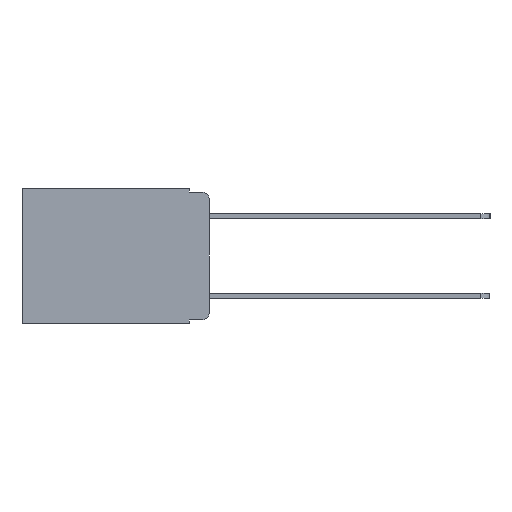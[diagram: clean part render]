
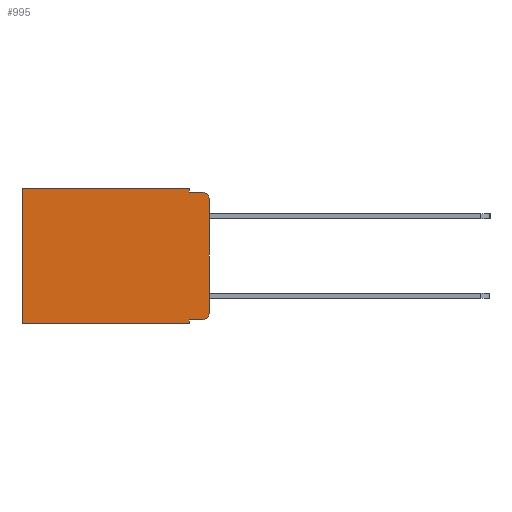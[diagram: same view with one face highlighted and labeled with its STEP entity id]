
A CAD part, left-side view. The second image highlights one B-rep face of the part: STEP entity #995.
In plain terms, the highlighted planar face has unit normal (-1, 0, 0).
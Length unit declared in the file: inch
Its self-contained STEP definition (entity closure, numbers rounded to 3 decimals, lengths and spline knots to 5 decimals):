
#72 = LINE ( 'NONE', #1308, #7037 ) ;
#288 = DIRECTION ( 'NONE',  ( 0., 0., -1. ) ) ;
#487 = CARTESIAN_POINT ( 'NONE',  ( 0.298, 0.051, 0. ) ) ;
#530 = VERTEX_POINT ( 'NONE', #7694 ) ;
#682 = CARTESIAN_POINT ( 'NONE',  ( 0.298, 0., -0.343 ) ) ;
#714 = VERTEX_POINT ( 'NONE', #6797 ) ;
#995 = ADVANCED_FACE ( 'NONE', ( #7935 ), #8241, .F. ) ;
#1308 = CARTESIAN_POINT ( 'NONE',  ( 0.298, 0.051, -0.333 ) ) ;
#1493 = VERTEX_POINT ( 'NONE', #7464 ) ;
#1528 = LINE ( 'NONE', #682, #12271 ) ;
#2037 = CARTESIAN_POINT ( 'NONE',  ( 0.298, 0.473, 0. ) ) ;
#2120 = VERTEX_POINT ( 'NONE', #9991 ) ;
#2572 = VECTOR ( 'NONE', #3281, 39.37008 ) ;
#2613 = CARTESIAN_POINT ( 'NONE',  ( 0.298, 0.02, -0.333 ) ) ;
#2808 = CARTESIAN_POINT ( 'NONE',  ( 0.298, 0.051, -0.01 ) ) ;
#3080 = CARTESIAN_POINT ( 'NONE',  ( 0.298, 0.473, 0. ) ) ;
#3187 = AXIS2_PLACEMENT_3D ( 'NONE', #6987, #13480, #288 ) ;
#3281 = DIRECTION ( 'NONE',  ( 0., 0., -1. ) ) ;
#3573 = AXIS2_PLACEMENT_3D ( 'NONE', #6587, #13032, #7615 ) ;
#3595 = VERTEX_POINT ( 'NONE', #12487 ) ;
#3895 = EDGE_LOOP ( 'NONE', ( #4255, #4319, #4393, #4439, #4554, #4566, #4617, #4631, #4651, #4721 ) ) ;
#4255 = ORIENTED_EDGE ( 'NONE', *, *, #13575, .F. ) ;
#4319 = ORIENTED_EDGE ( 'NONE', *, *, #12394, .T. ) ;
#4347 = DIRECTION ( 'NONE',  ( 0., 0., -1. ) ) ;
#4393 = ORIENTED_EDGE ( 'NONE', *, *, #11789, .F. ) ;
#4439 = ORIENTED_EDGE ( 'NONE', *, *, #11207, .F. ) ;
#4554 = ORIENTED_EDGE ( 'NONE', *, *, #8830, .T. ) ;
#4566 = ORIENTED_EDGE ( 'NONE', *, *, #10609, .T. ) ;
#4617 = ORIENTED_EDGE ( 'NONE', *, *, #13356, .F. ) ;
#4631 = ORIENTED_EDGE ( 'NONE', *, *, #8359, .F. ) ;
#4651 = ORIENTED_EDGE ( 'NONE', *, *, #7861, .T. ) ;
#4699 = DIRECTION ( 'NONE',  ( -1., 0., 0. ) ) ;
#4721 = ORIENTED_EDGE ( 'NONE', *, *, #7105, .T. ) ;
#4882 = VERTEX_POINT ( 'NONE', #2613 ) ;
#5200 = LINE ( 'NONE', #6043, #10101 ) ;
#5883 = VECTOR ( 'NONE', #8637, 39.37008 ) ;
#6043 = CARTESIAN_POINT ( 'NONE',  ( 0.298, 0., 0. ) ) ;
#6097 = CIRCLE ( 'NONE', #3573, 0.02 ) ;
#6587 = CARTESIAN_POINT ( 'NONE',  ( 0.298, 0.02, -0.313 ) ) ;
#6797 = CARTESIAN_POINT ( 'NONE',  ( 0.298, 0.473, -0.343 ) ) ;
#6987 = CARTESIAN_POINT ( 'NONE',  ( 0.298, 0., 0. ) ) ;
#7037 = VECTOR ( 'NONE', #9122, 39.37008 ) ;
#7070 = DIRECTION ( 'NONE',  ( 0., 1., 0. ) ) ;
#7105 = EDGE_CURVE ( 'NONE', #4882, #1493, #6097, .T. ) ;
#7294 = VECTOR ( 'NONE', #10048, 39.37008 ) ;
#7464 = CARTESIAN_POINT ( 'NONE',  ( 0.298, 0., -0.313 ) ) ;
#7615 = DIRECTION ( 'NONE',  ( 0., 0., -1. ) ) ;
#7694 = CARTESIAN_POINT ( 'NONE',  ( 0.298, 0.02, -0.01 ) ) ;
#7710 = CARTESIAN_POINT ( 'NONE',  ( 0.298, 0.051, 0. ) ) ;
#7861 = EDGE_CURVE ( 'NONE', #2120, #4882, #72, .T. ) ;
#7919 = LINE ( 'NONE', #3080, #12459 ) ;
#7935 = FACE_OUTER_BOUND ( 'NONE', #3895, .T. ) ;
#8177 = CARTESIAN_POINT ( 'NONE',  ( 0.298, 0., -0.03 ) ) ;
#8241 = PLANE ( 'NONE',  #3187 ) ;
#8359 = EDGE_CURVE ( 'NONE', #2120, #11293, #9669, .T. ) ;
#8601 = DIRECTION ( 'NONE',  ( 0., 0., -1. ) ) ;
#8610 = CIRCLE ( 'NONE', #12117, 0.02 ) ;
#8637 = DIRECTION ( 'NONE',  ( 0., 0., -1. ) ) ;
#8729 = LINE ( 'NONE', #9593, #2572 ) ;
#8830 = EDGE_CURVE ( 'NONE', #3595, #10005, #5200, .T. ) ;
#9122 = DIRECTION ( 'NONE',  ( 0., -1., 0. ) ) ;
#9593 = CARTESIAN_POINT ( 'NONE',  ( 0.298, 0., 0. ) ) ;
#9658 = DIRECTION ( 'NONE',  ( 0., 1., 0. ) ) ;
#9669 = LINE ( 'NONE', #487, #12335 ) ;
#9991 = CARTESIAN_POINT ( 'NONE',  ( 0.298, 0.051, -0.333 ) ) ;
#10005 = VERTEX_POINT ( 'NONE', #2037 ) ;
#10048 = DIRECTION ( 'NONE',  ( 0., -1., 0. ) ) ;
#10051 = LINE ( 'NONE', #10961, #7294 ) ;
#10101 = VECTOR ( 'NONE', #7070, 39.37008 ) ;
#10473 = VERTEX_POINT ( 'NONE', #2808 ) ;
#10561 = CARTESIAN_POINT ( 'NONE',  ( 0.298, 0.051, -0.343 ) ) ;
#10609 = EDGE_CURVE ( 'NONE', #10005, #714, #7919, .T. ) ;
#10637 = CARTESIAN_POINT ( 'NONE',  ( 0.298, 0.02, -0.03 ) ) ;
#10932 = LINE ( 'NONE', #7710, #5883 ) ;
#10961 = CARTESIAN_POINT ( 'NONE',  ( 0.298, 0.051, -0.01 ) ) ;
#11207 = EDGE_CURVE ( 'NONE', #3595, #10473, #10932, .T. ) ;
#11293 = VERTEX_POINT ( 'NONE', #10561 ) ;
#11522 = DIRECTION ( 'NONE',  ( 0., 0., -1. ) ) ;
#11789 = EDGE_CURVE ( 'NONE', #10473, #530, #10051, .T. ) ;
#12117 = AXIS2_PLACEMENT_3D ( 'NONE', #10637, #4699, #11522 ) ;
#12271 = VECTOR ( 'NONE', #9658, 39.37008 ) ;
#12335 = VECTOR ( 'NONE', #8601, 39.37008 ) ;
#12394 = EDGE_CURVE ( 'NONE', #12848, #530, #8610, .T. ) ;
#12459 = VECTOR ( 'NONE', #4347, 39.37008 ) ;
#12487 = CARTESIAN_POINT ( 'NONE',  ( 0.298, 0.051, 0. ) ) ;
#12848 = VERTEX_POINT ( 'NONE', #8177 ) ;
#13032 = DIRECTION ( 'NONE',  ( -1., 0., 0. ) ) ;
#13356 = EDGE_CURVE ( 'NONE', #11293, #714, #1528, .T. ) ;
#13480 = DIRECTION ( 'NONE',  ( 1., 0., 0. ) ) ;
#13575 = EDGE_CURVE ( 'NONE', #12848, #1493, #8729, .T. ) ;
